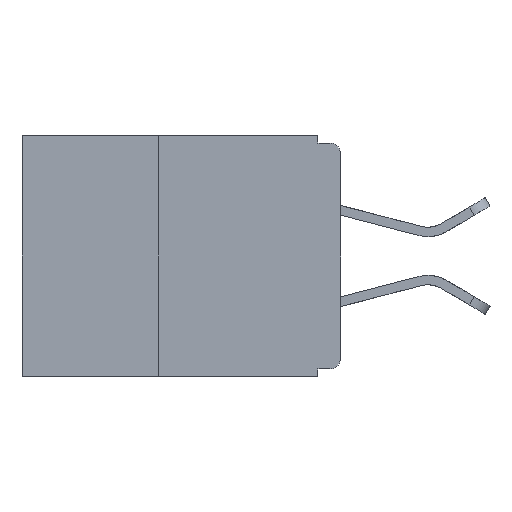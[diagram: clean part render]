
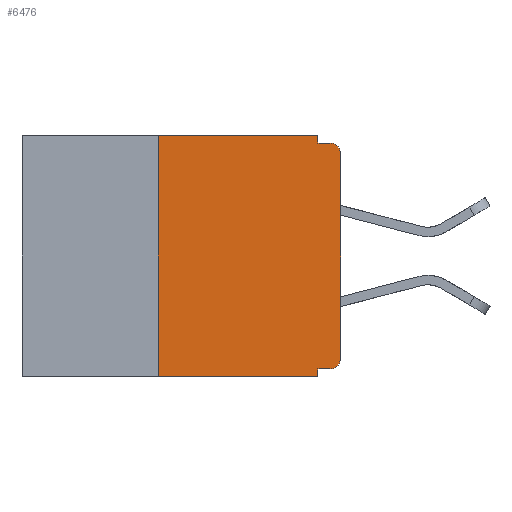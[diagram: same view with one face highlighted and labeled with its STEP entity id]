
A CAD part, left-side view. The second image highlights one B-rep face of the part: STEP entity #6476.
In plain terms, the highlighted planar face has unit normal (-1, 0, 0).
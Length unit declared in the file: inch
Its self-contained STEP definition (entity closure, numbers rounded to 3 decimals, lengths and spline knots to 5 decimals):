
#251 = LINE ( 'NONE', #1323, #17127 ) ;
#320 = ORIENTED_EDGE ( 'NONE', *, *, #4617, .F. ) ;
#916 = AXIS2_PLACEMENT_3D ( 'NONE', #11911, #5781, #1392 ) ;
#1017 = VECTOR ( 'NONE', #11291, 39.37008 ) ;
#1036 = VERTEX_POINT ( 'NONE', #4355 ) ;
#1323 = CARTESIAN_POINT ( 'NONE',  ( 0., 0.25, -0.33 ) ) ;
#1392 = DIRECTION ( 'NONE',  ( 0., 0., -1. ) ) ;
#1683 = ORIENTED_EDGE ( 'NONE', *, *, #4194, .F. ) ;
#1852 = VERTEX_POINT ( 'NONE', #2262 ) ;
#2052 = EDGE_CURVE ( 'NONE', #11378, #10418, #11161, .T. ) ;
#2138 = VECTOR ( 'NONE', #13913, 39.37008 ) ;
#2238 = LINE ( 'NONE', #3067, #15936 ) ;
#2262 = CARTESIAN_POINT ( 'NONE',  ( 0., 0.015, -0.01 ) ) ;
#2782 = VERTEX_POINT ( 'NONE', #10202 ) ;
#2992 = DIRECTION ( 'NONE',  ( 0., -1., 0. ) ) ;
#3014 = EDGE_CURVE ( 'NONE', #10418, #1852, #14353, .T. ) ;
#3067 = CARTESIAN_POINT ( 'NONE',  ( 0., 0.437, 0. ) ) ;
#3850 = VERTEX_POINT ( 'NONE', #7698 ) ;
#4131 = CARTESIAN_POINT ( 'NONE',  ( 0., 0.25, -0.33 ) ) ;
#4194 = EDGE_CURVE ( 'NONE', #9474, #1036, #2238, .T. ) ;
#4355 = CARTESIAN_POINT ( 'NONE',  ( 0., 0.031, 0. ) ) ;
#4528 = CARTESIAN_POINT ( 'NONE',  ( 0., 0.25, 0. ) ) ;
#4617 = EDGE_CURVE ( 'NONE', #13634, #9474, #251, .T. ) ;
#5104 = CARTESIAN_POINT ( 'NONE',  ( 0., 0., -0.01 ) ) ;
#5152 = VECTOR ( 'NONE', #8386, 39.37008 ) ;
#5598 = ORIENTED_EDGE ( 'NONE', *, *, #6329, .T. ) ;
#5781 = DIRECTION ( 'NONE',  ( -1., 0., 0. ) ) ;
#6329 = EDGE_CURVE ( 'NONE', #2782, #11378, #7887, .T. ) ;
#6476 = ADVANCED_FACE ( 'NONE', ( #12841 ), #15821, .F. ) ;
#7100 = CARTESIAN_POINT ( 'NONE',  ( 0., 0.437, -0.33 ) ) ;
#7219 = EDGE_CURVE ( 'NONE', #3850, #8768, #8230, .T. ) ;
#7227 = LINE ( 'NONE', #8956, #17242 ) ;
#7404 = ORIENTED_EDGE ( 'NONE', *, *, #15619, .F. ) ;
#7698 = CARTESIAN_POINT ( 'NONE',  ( 0., 0.031, -0.32 ) ) ;
#7887 = CIRCLE ( 'NONE', #17176, 0.015 ) ;
#8230 = LINE ( 'NONE', #11348, #1017 ) ;
#8386 = DIRECTION ( 'NONE',  ( 0., 0., 1. ) ) ;
#8653 = DIRECTION ( 'NONE',  ( 0., 0., 1. ) ) ;
#8768 = VERTEX_POINT ( 'NONE', #15271 ) ;
#8781 = VERTEX_POINT ( 'NONE', #14588 ) ;
#8956 = CARTESIAN_POINT ( 'NONE',  ( 0., 0., -0.32 ) ) ;
#9347 = LINE ( 'NONE', #12640, #2138 ) ;
#9474 = VERTEX_POINT ( 'NONE', #4528 ) ;
#9762 = VECTOR ( 'NONE', #14947, 39.37008 ) ;
#10202 = CARTESIAN_POINT ( 'NONE',  ( 0., 0.015, -0.32 ) ) ;
#10294 = DIRECTION ( 'NONE',  ( 0., 1., 0. ) ) ;
#10350 = CARTESIAN_POINT ( 'NONE',  ( 0., 0., 0. ) ) ;
#10366 = DIRECTION ( 'NONE',  ( 0., -1., 0. ) ) ;
#10418 = VERTEX_POINT ( 'NONE', #14285 ) ;
#10795 = EDGE_LOOP ( 'NONE', ( #14805, #15170, #7404, #11353, #1683, #320, #12432, #14176, #16961, #5598 ) ) ;
#11161 = LINE ( 'NONE', #10350, #5152 ) ;
#11203 = VECTOR ( 'NONE', #10366, 39.37008 ) ;
#11291 = DIRECTION ( 'NONE',  ( 0., 0., -1. ) ) ;
#11348 = CARTESIAN_POINT ( 'NONE',  ( 0., 0.031, -0.33 ) ) ;
#11353 = ORIENTED_EDGE ( 'NONE', *, *, #11405, .F. ) ;
#11378 = VERTEX_POINT ( 'NONE', #13636 ) ;
#11405 = EDGE_CURVE ( 'NONE', #1036, #8781, #9347, .T. ) ;
#11528 = EDGE_CURVE ( 'NONE', #2782, #3850, #7227, .T. ) ;
#11676 = AXIS2_PLACEMENT_3D ( 'NONE', #16197, #15295, #15175 ) ;
#11911 = CARTESIAN_POINT ( 'NONE',  ( 0., 0.015, -0.025 ) ) ;
#12432 = ORIENTED_EDGE ( 'NONE', *, *, #15917, .T. ) ;
#12640 = CARTESIAN_POINT ( 'NONE',  ( 0., 0.031, 0. ) ) ;
#12841 = FACE_OUTER_BOUND ( 'NONE', #10795, .T. ) ;
#13175 = DIRECTION ( 'NONE',  ( 0., 0., -1. ) ) ;
#13212 = LINE ( 'NONE', #7100, #9762 ) ;
#13561 = DIRECTION ( 'NONE',  ( -1., 0., 0. ) ) ;
#13634 = VERTEX_POINT ( 'NONE', #4131 ) ;
#13636 = CARTESIAN_POINT ( 'NONE',  ( 0., 0., -0.305 ) ) ;
#13794 = CARTESIAN_POINT ( 'NONE',  ( 0., 0.015, -0.305 ) ) ;
#13913 = DIRECTION ( 'NONE',  ( 0., 0., -1. ) ) ;
#14176 = ORIENTED_EDGE ( 'NONE', *, *, #7219, .F. ) ;
#14285 = CARTESIAN_POINT ( 'NONE',  ( 0., 0., -0.025 ) ) ;
#14353 = CIRCLE ( 'NONE', #916, 0.015 ) ;
#14588 = CARTESIAN_POINT ( 'NONE',  ( 0., 0.031, -0.01 ) ) ;
#14641 = LINE ( 'NONE', #5104, #11203 ) ;
#14805 = ORIENTED_EDGE ( 'NONE', *, *, #2052, .T. ) ;
#14947 = DIRECTION ( 'NONE',  ( 0., -1., 0. ) ) ;
#15170 = ORIENTED_EDGE ( 'NONE', *, *, #3014, .T. ) ;
#15175 = DIRECTION ( 'NONE',  ( 0., 0., -1. ) ) ;
#15271 = CARTESIAN_POINT ( 'NONE',  ( 0., 0.031, -0.33 ) ) ;
#15295 = DIRECTION ( 'NONE',  ( 1., 0., 0. ) ) ;
#15619 = EDGE_CURVE ( 'NONE', #8781, #1852, #14641, .T. ) ;
#15821 = PLANE ( 'NONE',  #11676 ) ;
#15917 = EDGE_CURVE ( 'NONE', #13634, #8768, #13212, .T. ) ;
#15936 = VECTOR ( 'NONE', #2992, 39.37008 ) ;
#16197 = CARTESIAN_POINT ( 'NONE',  ( 0., 0.437, 0. ) ) ;
#16961 = ORIENTED_EDGE ( 'NONE', *, *, #11528, .F. ) ;
#17127 = VECTOR ( 'NONE', #8653, 39.37008 ) ;
#17176 = AXIS2_PLACEMENT_3D ( 'NONE', #13794, #13561, #13175 ) ;
#17242 = VECTOR ( 'NONE', #10294, 39.37008 ) ;
